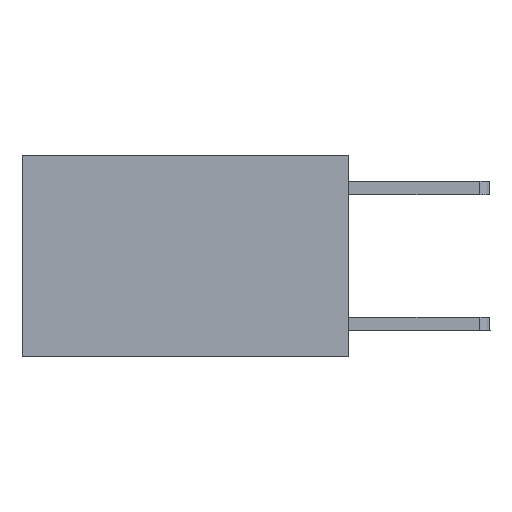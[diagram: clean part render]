
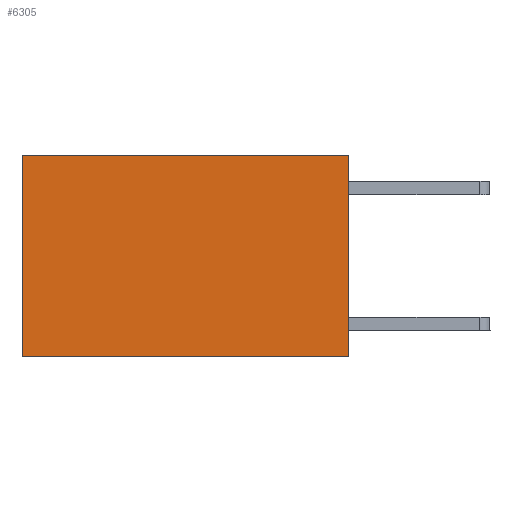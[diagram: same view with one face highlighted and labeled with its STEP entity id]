
A CAD part, left-side view. The second image highlights one B-rep face of the part: STEP entity #6305.
In plain terms, the highlighted planar face has unit normal (-1, 0, 0).
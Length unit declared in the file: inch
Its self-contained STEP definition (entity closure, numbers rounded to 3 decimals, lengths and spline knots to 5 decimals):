
#172 = VECTOR ( 'NONE', #9971, 39.37008 ) ;
#215 = LINE ( 'NONE', #6637, #172 ) ;
#622 = ORIENTED_EDGE ( 'NONE', *, *, #4723, .T. ) ;
#665 = ORIENTED_EDGE ( 'NONE', *, *, #8829, .F. ) ;
#678 = ORIENTED_EDGE ( 'NONE', *, *, #9855, .F. ) ;
#733 = ORIENTED_EDGE ( 'NONE', *, *, #1166, .T. ) ;
#757 = CARTESIAN_POINT ( 'NONE',  ( 0.2625, 0.6, 0. ) ) ;
#799 = CARTESIAN_POINT ( 'NONE',  ( 0.2625, 0.6, 0. ) ) ;
#1070 = CARTESIAN_POINT ( 'NONE',  ( 0.2625, 0., 0. ) ) ;
#1166 = EDGE_CURVE ( 'NONE', #8274, #8607, #215, .T. ) ;
#1221 = DIRECTION ( 'NONE',  ( 0., 0., -1. ) ) ;
#1352 = VECTOR ( 'NONE', #1974, 39.37008 ) ;
#1974 = DIRECTION ( 'NONE',  ( 0., 0., -1. ) ) ;
#2002 = VERTEX_POINT ( 'NONE', #3308 ) ;
#2474 = VECTOR ( 'NONE', #1221, 39.37008 ) ;
#2598 = CARTESIAN_POINT ( 'NONE',  ( 0.2625, 0., -0.37 ) ) ;
#2987 = LINE ( 'NONE', #799, #2474 ) ;
#3234 = CARTESIAN_POINT ( 'NONE',  ( 0.2625, 0.6, -0.37 ) ) ;
#3308 = CARTESIAN_POINT ( 'NONE',  ( 0.2625, 0., -0.37 ) ) ;
#3461 = LINE ( 'NONE', #8410, #1352 ) ;
#4210 = PLANE ( 'NONE',  #7429 ) ;
#4236 = DIRECTION ( 'NONE',  ( 0., 0., -1. ) ) ;
#4443 = LINE ( 'NONE', #2598, #8323 ) ;
#4723 = EDGE_CURVE ( 'NONE', #8607, #7942, #2987, .T. ) ;
#5254 = CARTESIAN_POINT ( 'NONE',  ( 0.2625, 0., 0. ) ) ;
#6305 = ADVANCED_FACE ( 'NONE', ( #8477 ), #4210, .F. ) ;
#6637 = CARTESIAN_POINT ( 'NONE',  ( 0.2625, 0., 0. ) ) ;
#7429 = AXIS2_PLACEMENT_3D ( 'NONE', #1070, #9091, #4236 ) ;
#7933 = EDGE_LOOP ( 'NONE', ( #622, #665, #678, #733 ) ) ;
#7942 = VERTEX_POINT ( 'NONE', #3234 ) ;
#8274 = VERTEX_POINT ( 'NONE', #5254 ) ;
#8323 = VECTOR ( 'NONE', #9018, 39.37008 ) ;
#8410 = CARTESIAN_POINT ( 'NONE',  ( 0.2625, 0., 0. ) ) ;
#8477 = FACE_OUTER_BOUND ( 'NONE', #7933, .T. ) ;
#8607 = VERTEX_POINT ( 'NONE', #757 ) ;
#8829 = EDGE_CURVE ( 'NONE', #2002, #7942, #4443, .T. ) ;
#9018 = DIRECTION ( 'NONE',  ( 0., 1., 0. ) ) ;
#9091 = DIRECTION ( 'NONE',  ( 1., 0., 0. ) ) ;
#9855 = EDGE_CURVE ( 'NONE', #8274, #2002, #3461, .T. ) ;
#9971 = DIRECTION ( 'NONE',  ( 0., 1., 0. ) ) ;
